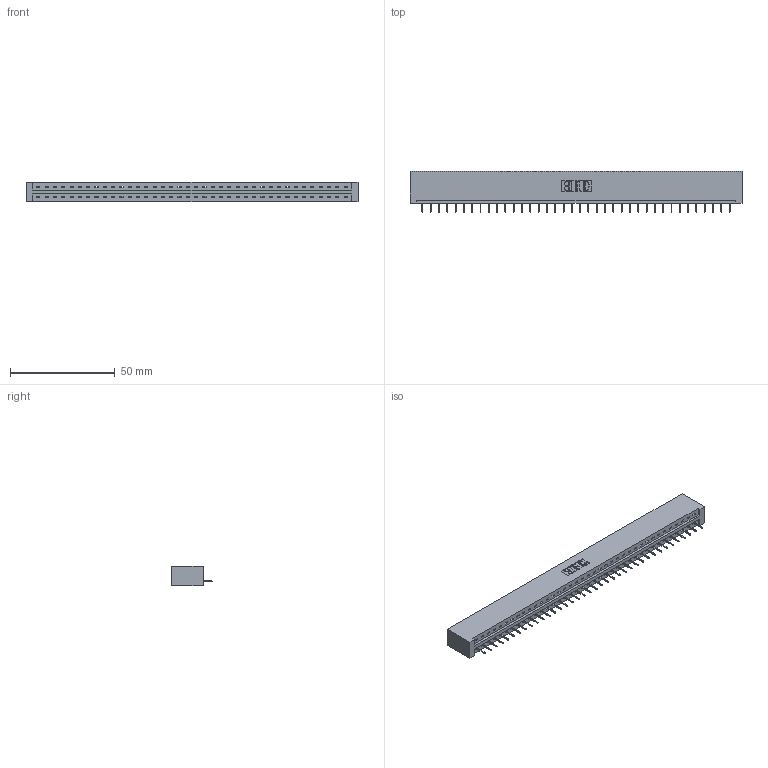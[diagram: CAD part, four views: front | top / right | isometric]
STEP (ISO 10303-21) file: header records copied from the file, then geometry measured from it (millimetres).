
FILE_DESCRIPTION (( 'STEP AP203' ), '1' );
FILE_NAME ('837-038-524-101.STEP', '2021-08-04T14:47:06', ( '' ), ( '' ), 'SwSTEP 2.0', 'SolidWorks 2020', '' );
FILE_SCHEMA (( 'CONFIG_CONTROL_DESIGN' ));
Length unit declared in the file: inch
Products named in the file (3): 837 Part_No Mounting Lugs; 837-038-524-101; 345-292-001_345-293-124
Assembly tree (39 placements, depth 2):
  837-038-524-101
    837 Part_No Mounting Lugs
    345-292-001_345-293-124  x38
Bounding box: 158.45 x 19.69 x 9.4 mm (x, y, z)
Volume: 17006.3 mm3; surface area: 17004.8 mm2
Topology: 39 solids, 39 shells, 2614 faces, 7583 edges, 4902 vertices
Faces by surface type: plane 2042, cylinder 572
Entity records: 28561 total; most frequent: CARTESIAN_POINT 4980, ORIENTED_EDGE 4954, DIRECTION 4193, EDGE_CURVE 2477, VECTOR 2361, LINE 2361, VERTEX_POINT 1646, AXIS2_PLACEMENT_3D 916
